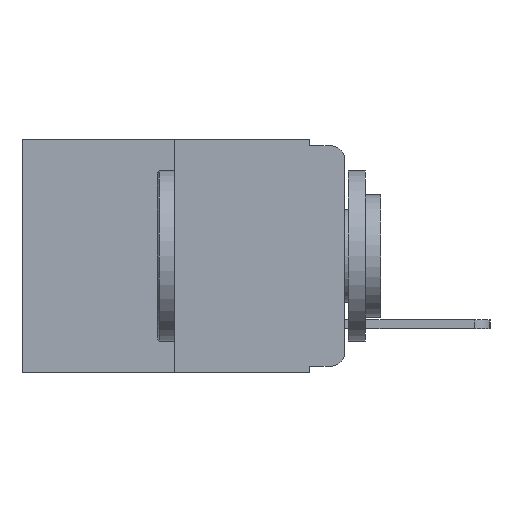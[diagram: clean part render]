
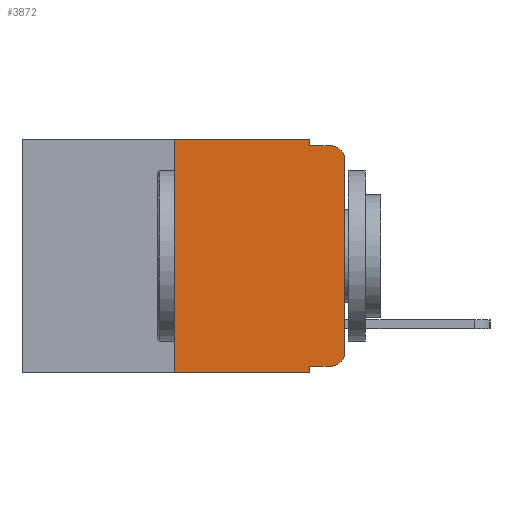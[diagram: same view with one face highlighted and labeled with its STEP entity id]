
A CAD part, left-side view. The second image highlights one B-rep face of the part: STEP entity #3872.
In plain terms, the highlighted planar face has unit normal (-1, 0, 0).
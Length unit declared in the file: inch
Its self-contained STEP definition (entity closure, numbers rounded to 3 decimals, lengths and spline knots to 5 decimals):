
#31 = CARTESIAN_POINT ( 'NONE',  ( 0., 0.02, -0.333 ) ) ;
#95 = VECTOR ( 'NONE', #9447, 39.37008 ) ;
#249 = CARTESIAN_POINT ( 'NONE',  ( 0., 0.051, -0.333 ) ) ;
#440 = CARTESIAN_POINT ( 'NONE',  ( 0., 0.051, 0. ) ) ;
#441 = ORIENTED_EDGE ( 'NONE', *, *, #8854, .T. ) ;
#491 = CIRCLE ( 'NONE', #872, 0.02 ) ;
#676 = VECTOR ( 'NONE', #9606, 39.37008 ) ;
#836 = VERTEX_POINT ( 'NONE', #952 ) ;
#872 = AXIS2_PLACEMENT_3D ( 'NONE', #11721, #5654, #12675 ) ;
#951 = EDGE_CURVE ( 'NONE', #1649, #9917, #11388, .T. ) ;
#952 = CARTESIAN_POINT ( 'NONE',  ( 0., 0.02, -0.01 ) ) ;
#1047 = VECTOR ( 'NONE', #6788, 39.37008 ) ;
#1329 = CARTESIAN_POINT ( 'NONE',  ( 0., 0.051, 0. ) ) ;
#1335 = VECTOR ( 'NONE', #2506, 39.37008 ) ;
#1347 = VECTOR ( 'NONE', #4850, 39.37008 ) ;
#1487 = CARTESIAN_POINT ( 'NONE',  ( 0., 0.25, -0.343 ) ) ;
#1567 = ORIENTED_EDGE ( 'NONE', *, *, #11578, .F. ) ;
#1601 = ORIENTED_EDGE ( 'NONE', *, *, #9565, .F. ) ;
#1649 = VERTEX_POINT ( 'NONE', #1806 ) ;
#1677 = VERTEX_POINT ( 'NONE', #1487 ) ;
#1806 = CARTESIAN_POINT ( 'NONE',  ( 0., 0., -0.313 ) ) ;
#1843 = CARTESIAN_POINT ( 'NONE',  ( 0., 0.25, 0. ) ) ;
#1844 = VECTOR ( 'NONE', #4059, 39.37008 ) ;
#2355 = CARTESIAN_POINT ( 'NONE',  ( 0., 0.051, -0.343 ) ) ;
#2506 = DIRECTION ( 'NONE',  ( 0., -1., 0. ) ) ;
#2791 = VECTOR ( 'NONE', #3968, 39.37008 ) ;
#2856 = DIRECTION ( 'NONE',  ( 0., 0., 1. ) ) ;
#3872 = ADVANCED_FACE ( 'NONE', ( #13106 ), #12649, .F. ) ;
#3968 = DIRECTION ( 'NONE',  ( 0., -1., 0. ) ) ;
#4041 = VERTEX_POINT ( 'NONE', #249 ) ;
#4059 = DIRECTION ( 'NONE',  ( 0., 0., -1. ) ) ;
#4494 = LINE ( 'NONE', #11918, #1347 ) ;
#4617 = LINE ( 'NONE', #11191, #1844 ) ;
#4669 = VERTEX_POINT ( 'NONE', #5281 ) ;
#4816 = CARTESIAN_POINT ( 'NONE',  ( 0., 0., 0. ) ) ;
#4850 = DIRECTION ( 'NONE',  ( 0., -1., 0. ) ) ;
#5005 = ORIENTED_EDGE ( 'NONE', *, *, #9481, .T. ) ;
#5064 = CARTESIAN_POINT ( 'NONE',  ( 0., 0.02, -0.03 ) ) ;
#5259 = VERTEX_POINT ( 'NONE', #2355 ) ;
#5281 = CARTESIAN_POINT ( 'NONE',  ( 0., 0.051, -0.01 ) ) ;
#5581 = LINE ( 'NONE', #7002, #2791 ) ;
#5603 = CARTESIAN_POINT ( 'NONE',  ( 0., 0.051, -0.333 ) ) ;
#5654 = DIRECTION ( 'NONE',  ( -1., 0., 0. ) ) ;
#5820 = LINE ( 'NONE', #11472, #95 ) ;
#5987 = EDGE_CURVE ( 'NONE', #8375, #8313, #4494, .T. ) ;
#6058 = DIRECTION ( 'NONE',  ( 0., 0., -1. ) ) ;
#6338 = DIRECTION ( 'NONE',  ( 1., 0., 0. ) ) ;
#6788 = DIRECTION ( 'NONE',  ( 0., 0., 1. ) ) ;
#7002 = CARTESIAN_POINT ( 'NONE',  ( 0., 0.473, -0.343 ) ) ;
#7094 = ORIENTED_EDGE ( 'NONE', *, *, #8221, .T. ) ;
#7599 = CARTESIAN_POINT ( 'NONE',  ( 0., 0., -0.03 ) ) ;
#7664 = AXIS2_PLACEMENT_3D ( 'NONE', #5064, #12112, #6058 ) ;
#8221 = EDGE_CURVE ( 'NONE', #9874, #1649, #491, .T. ) ;
#8267 = LINE ( 'NONE', #1843, #11255 ) ;
#8288 = EDGE_LOOP ( 'NONE', ( #9522, #11023, #9042, #1567, #10769, #9928, #5005, #1601, #441, #7094 ) ) ;
#8313 = VERTEX_POINT ( 'NONE', #440 ) ;
#8375 = VERTEX_POINT ( 'NONE', #10007 ) ;
#8854 = EDGE_CURVE ( 'NONE', #4041, #9874, #12220, .T. ) ;
#9042 = ORIENTED_EDGE ( 'NONE', *, *, #12235, .F. ) ;
#9186 = CARTESIAN_POINT ( 'NONE',  ( 0., 0.473, 0. ) ) ;
#9447 = DIRECTION ( 'NONE',  ( 0., -1., 0. ) ) ;
#9481 = EDGE_CURVE ( 'NONE', #1677, #5259, #5581, .T. ) ;
#9522 = ORIENTED_EDGE ( 'NONE', *, *, #951, .T. ) ;
#9565 = EDGE_CURVE ( 'NONE', #4041, #5259, #4617, .T. ) ;
#9606 = DIRECTION ( 'NONE',  ( 0., 0., -1. ) ) ;
#9650 = CIRCLE ( 'NONE', #7664, 0.02 ) ;
#9712 = AXIS2_PLACEMENT_3D ( 'NONE', #9186, #6338, #11591 ) ;
#9874 = VERTEX_POINT ( 'NONE', #31 ) ;
#9917 = VERTEX_POINT ( 'NONE', #7599 ) ;
#9928 = ORIENTED_EDGE ( 'NONE', *, *, #10925, .F. ) ;
#10007 = CARTESIAN_POINT ( 'NONE',  ( 0., 0.25, 0. ) ) ;
#10769 = ORIENTED_EDGE ( 'NONE', *, *, #5987, .F. ) ;
#10925 = EDGE_CURVE ( 'NONE', #1677, #8375, #8267, .T. ) ;
#11023 = ORIENTED_EDGE ( 'NONE', *, *, #12840, .T. ) ;
#11191 = CARTESIAN_POINT ( 'NONE',  ( 0., 0.051, 0. ) ) ;
#11255 = VECTOR ( 'NONE', #2856, 39.37008 ) ;
#11388 = LINE ( 'NONE', #4816, #1047 ) ;
#11472 = CARTESIAN_POINT ( 'NONE',  ( 0., 0.051, -0.01 ) ) ;
#11578 = EDGE_CURVE ( 'NONE', #8313, #4669, #11692, .T. ) ;
#11591 = DIRECTION ( 'NONE',  ( 0., 0., -1. ) ) ;
#11692 = LINE ( 'NONE', #1329, #676 ) ;
#11721 = CARTESIAN_POINT ( 'NONE',  ( 0., 0.02, -0.313 ) ) ;
#11918 = CARTESIAN_POINT ( 'NONE',  ( 0., 0.473, 0. ) ) ;
#12112 = DIRECTION ( 'NONE',  ( -1., 0., 0. ) ) ;
#12220 = LINE ( 'NONE', #5603, #1335 ) ;
#12235 = EDGE_CURVE ( 'NONE', #4669, #836, #5820, .T. ) ;
#12649 = PLANE ( 'NONE',  #9712 ) ;
#12675 = DIRECTION ( 'NONE',  ( 0., 0., -1. ) ) ;
#12840 = EDGE_CURVE ( 'NONE', #9917, #836, #9650, .T. ) ;
#13106 = FACE_OUTER_BOUND ( 'NONE', #8288, .T. ) ;
